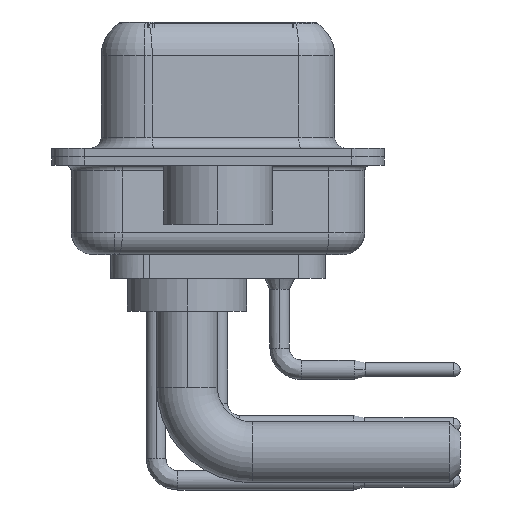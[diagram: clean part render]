
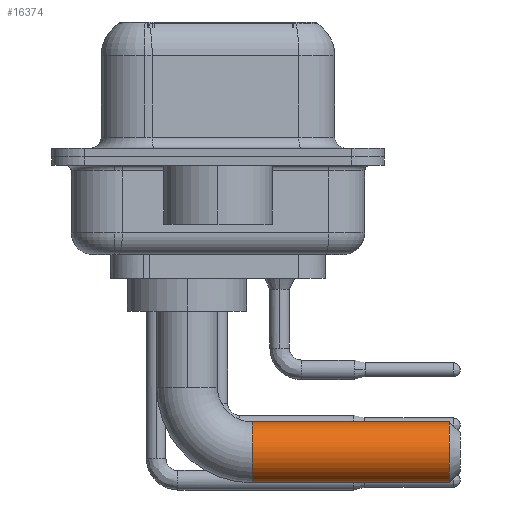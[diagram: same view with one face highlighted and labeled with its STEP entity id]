
A CAD part, left-side view. The second image highlights one B-rep face of the part: STEP entity #16374.
In plain terms, the highlighted cylindrical face has radius 1.4 mm (diameter 2.8 mm), a partial arc.
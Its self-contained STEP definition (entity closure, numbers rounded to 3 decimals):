
#151 = CARTESIAN_POINT ( 'NONE',  ( 0., -12.07, -7.9 ) ) ;
#1406 = AXIS2_PLACEMENT_3D ( 'NONE', #17963, #21714, #20338 ) ;
#4239 = EDGE_LOOP ( 'NONE', ( #12631, #5715, #6235, #15817 ) ) ;
#4598 = VECTOR ( 'NONE', #14038, 1000. ) ;
#4835 = EDGE_CURVE ( 'NONE', #5983, #21573, #7205, .T. ) ;
#5715 = ORIENTED_EDGE ( 'NONE', *, *, #16432, .T. ) ;
#5983 = VERTEX_POINT ( 'NONE', #21749 ) ;
#6235 = ORIENTED_EDGE ( 'NONE', *, *, #4835, .T. ) ;
#6718 = EDGE_CURVE ( 'NONE', #11405, #18922, #14577, .T. ) ;
#7205 = LINE ( 'NONE', #27203, #4598 ) ;
#7846 = FACE_OUTER_BOUND ( 'NONE', #4239, .T. ) ;
#8111 = CIRCLE ( 'NONE', #12864, 1.4 ) ;
#8301 = DIRECTION ( 'NONE',  ( 0., -1., 0. ) ) ;
#8714 = CARTESIAN_POINT ( 'NONE',  ( 0., -3., -5.1 ) ) ;
#10523 = DIRECTION ( 'NONE',  ( 0., 0., -1. ) ) ;
#11405 = VERTEX_POINT ( 'NONE', #8714 ) ;
#11662 = DIRECTION ( 'NONE',  ( -1., 0., 0. ) ) ;
#12631 = ORIENTED_EDGE ( 'NONE', *, *, #6718, .F. ) ;
#12864 = AXIS2_PLACEMENT_3D ( 'NONE', #24151, #18028, #11662 ) ;
#14038 = DIRECTION ( 'NONE',  ( 0., -1., 0. ) ) ;
#14577 = LINE ( 'NONE', #16955, #24509 ) ;
#15817 = ORIENTED_EDGE ( 'NONE', *, *, #27742, .T. ) ;
#16374 = ADVANCED_FACE ( 'NONE', ( #7846 ), #19120, .T. ) ;
#16432 = EDGE_CURVE ( 'NONE', #11405, #5983, #8111, .T. ) ;
#16955 = CARTESIAN_POINT ( 'NONE',  ( 0., -3., -5.1 ) ) ;
#17536 = CIRCLE ( 'NONE', #1406, 1.4 ) ;
#17963 = CARTESIAN_POINT ( 'NONE',  ( 0., -12.07, -6.5 ) ) ;
#18028 = DIRECTION ( 'NONE',  ( 0., -1., 0. ) ) ;
#18922 = VERTEX_POINT ( 'NONE', #26525 ) ;
#19120 = CYLINDRICAL_SURFACE ( 'NONE', #26056, 1.4 ) ;
#20338 = DIRECTION ( 'NONE',  ( 0., 0., -1. ) ) ;
#21573 = VERTEX_POINT ( 'NONE', #151 ) ;
#21714 = DIRECTION ( 'NONE',  ( 0., 1., 0. ) ) ;
#21749 = CARTESIAN_POINT ( 'NONE',  ( 0., -3., -7.9 ) ) ;
#24151 = CARTESIAN_POINT ( 'NONE',  ( 0., -3., -6.5 ) ) ;
#24509 = VECTOR ( 'NONE', #25831, 1000. ) ;
#25831 = DIRECTION ( 'NONE',  ( 0., -1., 0. ) ) ;
#26056 = AXIS2_PLACEMENT_3D ( 'NONE', #28136, #8301, #10523 ) ;
#26525 = CARTESIAN_POINT ( 'NONE',  ( 0., -12.07, -5.1 ) ) ;
#27203 = CARTESIAN_POINT ( 'NONE',  ( 0., -3., -7.9 ) ) ;
#27742 = EDGE_CURVE ( 'NONE', #21573, #18922, #17536, .T. ) ;
#28136 = CARTESIAN_POINT ( 'NONE',  ( 0., -3., -6.5 ) ) ;
